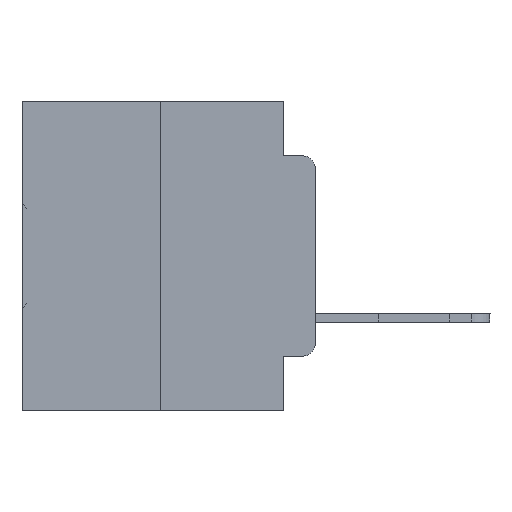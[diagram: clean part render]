
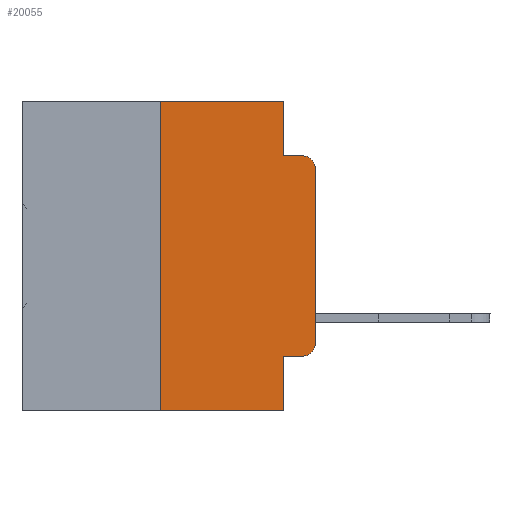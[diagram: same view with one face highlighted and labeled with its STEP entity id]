
A CAD part, left-side view. The second image highlights one B-rep face of the part: STEP entity #20055.
In plain terms, the highlighted planar face has unit normal (-1, 0, 0).
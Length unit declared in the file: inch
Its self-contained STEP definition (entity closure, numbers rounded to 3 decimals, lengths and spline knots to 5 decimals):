
#212 = ORIENTED_EDGE ( 'NONE', *, *, #28705, .T. ) ;
#714 = CARTESIAN_POINT ( 'NONE',  ( 0., 0.02, -0.0885 ) ) ;
#848 = VECTOR ( 'NONE', #28251, 39.37008 ) ;
#1294 = ORIENTED_EDGE ( 'NONE', *, *, #4833, .F. ) ;
#1745 = CARTESIAN_POINT ( 'NONE',  ( 0., 0.25, 0. ) ) ;
#1849 = CARTESIAN_POINT ( 'NONE',  ( 0., 0.25, -0.5 ) ) ;
#2165 = VECTOR ( 'NONE', #17631, 39.37008 ) ;
#2222 = DIRECTION ( 'NONE',  ( 0., 0., -1. ) ) ;
#2595 = DIRECTION ( 'NONE',  ( 1., 0., 0. ) ) ;
#3313 = DIRECTION ( 'NONE',  ( -1., 0., 0. ) ) ;
#3701 = CARTESIAN_POINT ( 'NONE',  ( 0., 0.02, -0.4115 ) ) ;
#4596 = CARTESIAN_POINT ( 'NONE',  ( 0., 0.473, 0. ) ) ;
#4647 = ORIENTED_EDGE ( 'NONE', *, *, #29266, .F. ) ;
#4833 = EDGE_CURVE ( 'NONE', #10235, #16720, #17702, .T. ) ;
#5413 = DIRECTION ( 'NONE',  ( 0., 0., -1. ) ) ;
#5723 = AXIS2_PLACEMENT_3D ( 'NONE', #22385, #6269, #27411 ) ;
#5849 = CARTESIAN_POINT ( 'NONE',  ( 0., 0.051, 0. ) ) ;
#6269 = DIRECTION ( 'NONE',  ( -1., 0., 0. ) ) ;
#6338 = EDGE_CURVE ( 'NONE', #18058, #15646, #18628, .T. ) ;
#6463 = VERTEX_POINT ( 'NONE', #10940 ) ;
#6888 = EDGE_CURVE ( 'NONE', #9167, #22687, #11020, .T. ) ;
#7053 = DIRECTION ( 'NONE',  ( 0., -1., 0. ) ) ;
#9167 = VERTEX_POINT ( 'NONE', #16571 ) ;
#9645 = DIRECTION ( 'NONE',  ( 0., -1., 0. ) ) ;
#10140 = EDGE_CURVE ( 'NONE', #15830, #18058, #12589, .T. ) ;
#10204 = EDGE_CURVE ( 'NONE', #15646, #19249, #20047, .T. ) ;
#10235 = VERTEX_POINT ( 'NONE', #1849 ) ;
#10253 = AXIS2_PLACEMENT_3D ( 'NONE', #16124, #2595, #13161 ) ;
#10940 = CARTESIAN_POINT ( 'NONE',  ( 0., 0.051, 0. ) ) ;
#11020 = LINE ( 'NONE', #21604, #28058 ) ;
#12184 = VECTOR ( 'NONE', #7053, 39.37008 ) ;
#12416 = VECTOR ( 'NONE', #2222, 39.37008 ) ;
#12507 = EDGE_CURVE ( 'NONE', #10235, #32703, #20228, .T. ) ;
#12589 = LINE ( 'NONE', #23153, #2165 ) ;
#13161 = DIRECTION ( 'NONE',  ( 0., 0., -1. ) ) ;
#13970 = ORIENTED_EDGE ( 'NONE', *, *, #6338, .T. ) ;
#14121 = CARTESIAN_POINT ( 'NONE',  ( 0., 0., -0.1085 ) ) ;
#14377 = VECTOR ( 'NONE', #22982, 39.37008 ) ;
#14763 = AXIS2_PLACEMENT_3D ( 'NONE', #18411, #3313, #5413 ) ;
#15646 = VERTEX_POINT ( 'NONE', #27161 ) ;
#15696 = EDGE_CURVE ( 'NONE', #6463, #9167, #32525, .T. ) ;
#15795 = PLANE ( 'NONE',  #10253 ) ;
#15830 = VERTEX_POINT ( 'NONE', #17298 ) ;
#16124 = CARTESIAN_POINT ( 'NONE',  ( 0., 0.473, 0. ) ) ;
#16571 = CARTESIAN_POINT ( 'NONE',  ( 0., 0.051, -0.0885 ) ) ;
#16720 = VERTEX_POINT ( 'NONE', #18345 ) ;
#16939 = ORIENTED_EDGE ( 'NONE', *, *, #24883, .F. ) ;
#17298 = CARTESIAN_POINT ( 'NONE',  ( 0., 0.051, -0.4115 ) ) ;
#17304 = ORIENTED_EDGE ( 'NONE', *, *, #10204, .T. ) ;
#17631 = DIRECTION ( 'NONE',  ( 0., -1., 0. ) ) ;
#17702 = LINE ( 'NONE', #1745, #848 ) ;
#18058 = VERTEX_POINT ( 'NONE', #3701 ) ;
#18345 = CARTESIAN_POINT ( 'NONE',  ( 0., 0.25, 0. ) ) ;
#18411 = CARTESIAN_POINT ( 'NONE',  ( 0., 0.02, -0.3915 ) ) ;
#18628 = CIRCLE ( 'NONE', #14763, 0.02 ) ;
#18701 = FACE_OUTER_BOUND ( 'NONE', #23847, .T. ) ;
#19249 = VERTEX_POINT ( 'NONE', #14121 ) ;
#19536 = ORIENTED_EDGE ( 'NONE', *, *, #12507, .T. ) ;
#20047 = LINE ( 'NONE', #25919, #14377 ) ;
#20055 = ADVANCED_FACE ( 'NONE', ( #18701 ), #15795, .F. ) ;
#20228 = LINE ( 'NONE', #30784, #12184 ) ;
#20597 = CARTESIAN_POINT ( 'NONE',  ( 0., 0.051, 0. ) ) ;
#21095 = VECTOR ( 'NONE', #9645, 39.37008 ) ;
#21604 = CARTESIAN_POINT ( 'NONE',  ( 0., 0.051, -0.0885 ) ) ;
#22385 = CARTESIAN_POINT ( 'NONE',  ( 0., 0.02, -0.1085 ) ) ;
#22687 = VERTEX_POINT ( 'NONE', #714 ) ;
#22982 = DIRECTION ( 'NONE',  ( 0., 0., 1. ) ) ;
#23020 = LINE ( 'NONE', #20597, #12416 ) ;
#23153 = CARTESIAN_POINT ( 'NONE',  ( 0., 0.051, -0.4115 ) ) ;
#23847 = EDGE_LOOP ( 'NONE', ( #17304, #212, #28702, #29035, #16939, #1294, #19536, #4647, #32205, #13970 ) ) ;
#23873 = DIRECTION ( 'NONE',  ( 0., 0., -1. ) ) ;
#24883 = EDGE_CURVE ( 'NONE', #16720, #6463, #27830, .T. ) ;
#25045 = VECTOR ( 'NONE', #23873, 39.37008 ) ;
#25919 = CARTESIAN_POINT ( 'NONE',  ( 0., 0., 0. ) ) ;
#27161 = CARTESIAN_POINT ( 'NONE',  ( 0., 0., -0.3915 ) ) ;
#27411 = DIRECTION ( 'NONE',  ( 0., 0., -1. ) ) ;
#27830 = LINE ( 'NONE', #4596, #21095 ) ;
#28058 = VECTOR ( 'NONE', #32153, 39.37008 ) ;
#28181 = CARTESIAN_POINT ( 'NONE',  ( 0., 0.051, -0.5 ) ) ;
#28251 = DIRECTION ( 'NONE',  ( 0., 0., 1. ) ) ;
#28702 = ORIENTED_EDGE ( 'NONE', *, *, #6888, .F. ) ;
#28705 = EDGE_CURVE ( 'NONE', #19249, #22687, #31177, .T. ) ;
#29035 = ORIENTED_EDGE ( 'NONE', *, *, #15696, .F. ) ;
#29266 = EDGE_CURVE ( 'NONE', #15830, #32703, #23020, .T. ) ;
#30784 = CARTESIAN_POINT ( 'NONE',  ( 0., 0.473, -0.5 ) ) ;
#31177 = CIRCLE ( 'NONE', #5723, 0.02 ) ;
#32153 = DIRECTION ( 'NONE',  ( 0., -1., 0. ) ) ;
#32205 = ORIENTED_EDGE ( 'NONE', *, *, #10140, .T. ) ;
#32525 = LINE ( 'NONE', #5849, #25045 ) ;
#32703 = VERTEX_POINT ( 'NONE', #28181 ) ;
